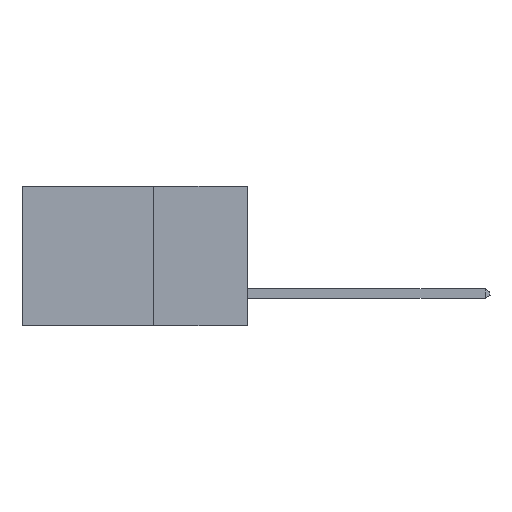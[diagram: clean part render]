
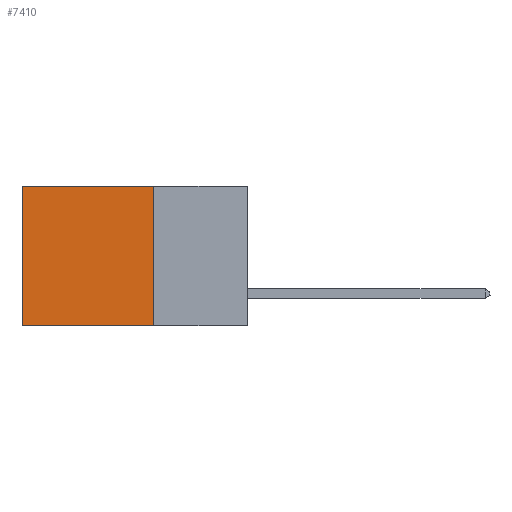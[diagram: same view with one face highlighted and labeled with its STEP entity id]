
A CAD part, left-side view. The second image highlights one B-rep face of the part: STEP entity #7410.
In plain terms, the highlighted planar face has unit normal (-1, 0, 0).
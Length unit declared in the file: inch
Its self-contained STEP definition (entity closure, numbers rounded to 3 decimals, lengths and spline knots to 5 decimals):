
#604 = VERTEX_POINT ( 'NONE', #19262 ) ;
#632 = EDGE_LOOP ( 'NONE', ( #14580, #15471, #21193, #22487 ) ) ;
#948 = VERTEX_POINT ( 'NONE', #11374 ) ;
#3454 = VECTOR ( 'NONE', #5794, 39.37008 ) ;
#4064 = LINE ( 'NONE', #6276, #10790 ) ;
#4952 = DIRECTION ( 'NONE',  ( 0., 0., -1. ) ) ;
#4979 = CARTESIAN_POINT ( 'NONE',  ( 0.298, 0.6, -0.37 ) ) ;
#5129 = EDGE_CURVE ( 'NONE', #948, #604, #4064, .T. ) ;
#5404 = CARTESIAN_POINT ( 'NONE',  ( 0.298, 0.25, 0. ) ) ;
#5794 = DIRECTION ( 'NONE',  ( 0., 1., 0. ) ) ;
#5974 = VERTEX_POINT ( 'NONE', #4979 ) ;
#6276 = CARTESIAN_POINT ( 'NONE',  ( 0.298, 0.25, 0. ) ) ;
#6749 = FACE_OUTER_BOUND ( 'NONE', #632, .T. ) ;
#7237 = LINE ( 'NONE', #14911, #16481 ) ;
#7410 = ADVANCED_FACE ( 'NONE', ( #6749 ), #19376, .F. ) ;
#8214 = EDGE_CURVE ( 'NONE', #948, #21426, #15140, .T. ) ;
#8770 = LINE ( 'NONE', #20084, #3454 ) ;
#8993 = DIRECTION ( 'NONE',  ( 0., 0., -1. ) ) ;
#9305 = DIRECTION ( 'NONE',  ( 0., 0., -1. ) ) ;
#10181 = DIRECTION ( 'NONE',  ( 1., 0., 0. ) ) ;
#10790 = VECTOR ( 'NONE', #18829, 39.37008 ) ;
#11374 = CARTESIAN_POINT ( 'NONE',  ( 0.298, 0.25, 0. ) ) ;
#13965 = CARTESIAN_POINT ( 'NONE',  ( 0.298, 0.25, 0. ) ) ;
#14580 = ORIENTED_EDGE ( 'NONE', *, *, #15573, .T. ) ;
#14911 = CARTESIAN_POINT ( 'NONE',  ( 0.298, 0.6, 0. ) ) ;
#15140 = LINE ( 'NONE', #5404, #15691 ) ;
#15471 = ORIENTED_EDGE ( 'NONE', *, *, #21355, .F. ) ;
#15573 = EDGE_CURVE ( 'NONE', #604, #5974, #7237, .T. ) ;
#15691 = VECTOR ( 'NONE', #8993, 39.37008 ) ;
#16481 = VECTOR ( 'NONE', #9305, 39.37008 ) ;
#18829 = DIRECTION ( 'NONE',  ( 0., 1., 0. ) ) ;
#19262 = CARTESIAN_POINT ( 'NONE',  ( 0.298, 0.6, 0. ) ) ;
#19376 = PLANE ( 'NONE',  #19694 ) ;
#19694 = AXIS2_PLACEMENT_3D ( 'NONE', #13965, #10181, #4952 ) ;
#20084 = CARTESIAN_POINT ( 'NONE',  ( 0.298, 0.25, -0.37 ) ) ;
#20471 = CARTESIAN_POINT ( 'NONE',  ( 0.298, 0.25, -0.37 ) ) ;
#21193 = ORIENTED_EDGE ( 'NONE', *, *, #8214, .F. ) ;
#21355 = EDGE_CURVE ( 'NONE', #21426, #5974, #8770, .T. ) ;
#21426 = VERTEX_POINT ( 'NONE', #20471 ) ;
#22487 = ORIENTED_EDGE ( 'NONE', *, *, #5129, .T. ) ;
